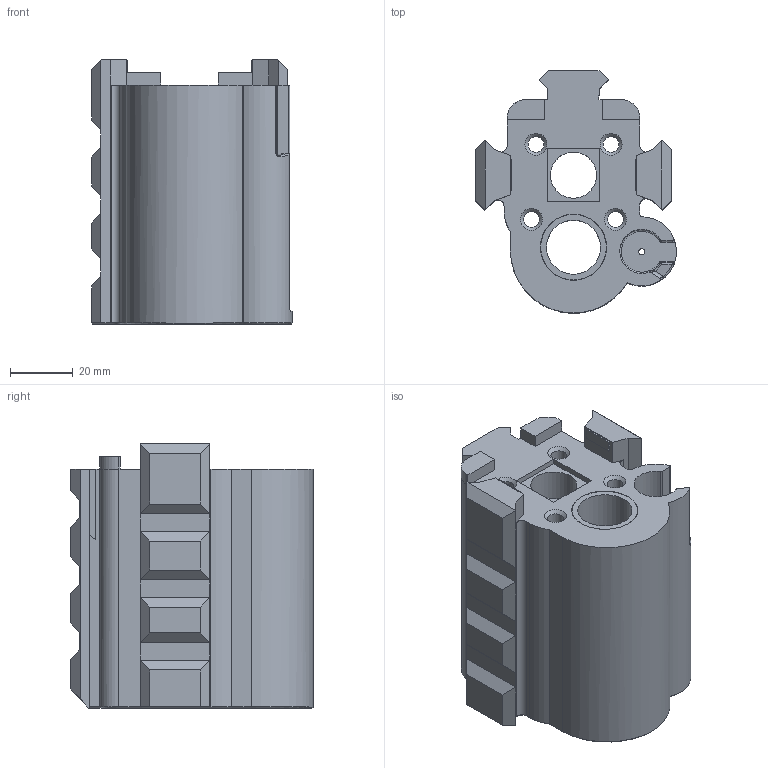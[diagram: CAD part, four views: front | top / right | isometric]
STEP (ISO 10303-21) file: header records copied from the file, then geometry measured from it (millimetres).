
FILE_DESCRIPTION (( 'STEP AP203' ), '1' );
FILE_NAME ('WTF-9H_barrel_retainer.STEP', '2020-06-09T21:42:43', ( '' ), ( '' ), 'SwSTEP 2.0', 'SolidWorks 2016', '' );
FILE_SCHEMA (( 'CONFIG_CONTROL_DESIGN' ));
Length unit declared in the file: millimetre
Products named in the file (1): WTF-9H_barrel_retainer
Bounding box: 63.85 x 77.09 x 84.02 mm (x, y, z)
Volume: 153539 mm3; surface area: 43000.8 mm2
Topology: 1 solids, 1 shells, 259 faces, 675 edges, 422 vertices
Faces by surface type: plane 169, cylinder 47, cone 31, bspline 12
Full cylindrical faces by diameter (mm): 2 x1, 5 x4, 14.7 x1, 17.2 x1
Entity records: 8312 total; most frequent: CARTESIAN_POINT 2094, ORIENTED_EDGE 1304, DIRECTION 1194, EDGE_CURVE 652, LINE 472, VECTOR 472, VERTEX_POINT 413, AXIS2_PLACEMENT_3D 361
